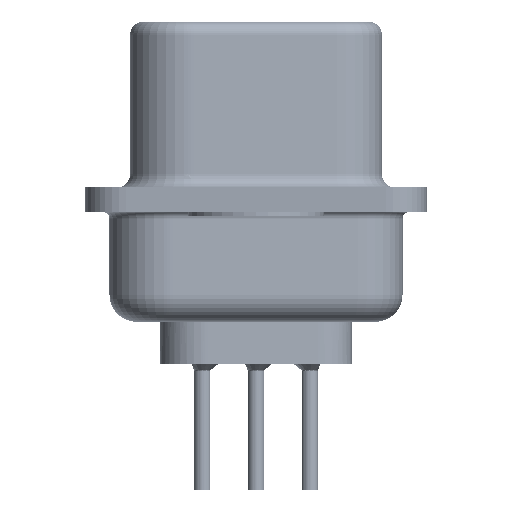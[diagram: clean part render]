
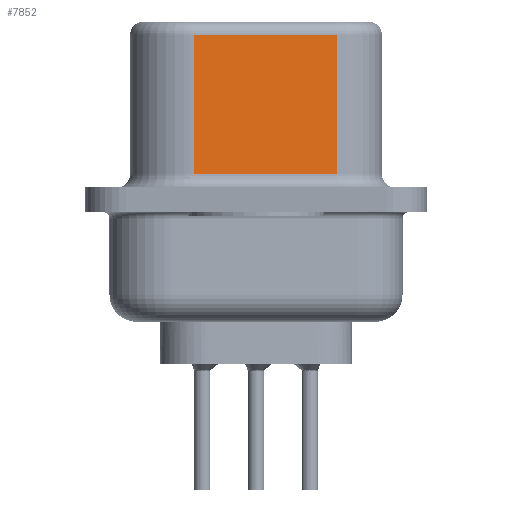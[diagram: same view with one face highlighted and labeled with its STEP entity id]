
A CAD part, left-side view. The second image highlights one B-rep face of the part: STEP entity #7852.
In plain terms, the highlighted planar face has unit normal (-0.985, -0.174, 0).
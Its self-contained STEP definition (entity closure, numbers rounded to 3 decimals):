
#1953 = DIRECTION ( 'NONE',  ( 0., 0., -1. ) ) ;
#3079 = CARTESIAN_POINT ( 'NONE',  ( 4.551, -2.987, 6.07 ) ) ;
#3446 = CARTESIAN_POINT ( 'NONE',  ( 4.551, -2.987, 0.95 ) ) ;
#3955 = LINE ( 'NONE', #13859, #12807 ) ;
#5753 = EDGE_CURVE ( 'NONE', #15745, #7015, #3955, .T. ) ;
#7015 = VERTEX_POINT ( 'NONE', #27484 ) ;
#7018 = ORIENTED_EDGE ( 'NONE', *, *, #5753, .T. ) ;
#7852 = ADVANCED_FACE ( 'NONE', ( #9505 ), #21688, .F. ) ;
#8323 = EDGE_CURVE ( 'NONE', #18790, #12468, #19392, .T. ) ;
#9505 = FACE_OUTER_BOUND ( 'NONE', #10460, .T. ) ;
#9689 = ORIENTED_EDGE ( 'NONE', *, *, #16191, .T. ) ;
#10460 = EDGE_LOOP ( 'NONE', ( #18000, #9689, #7018, #23546 ) ) ;
#11807 = VECTOR ( 'NONE', #1953, 1000. ) ;
#12468 = VERTEX_POINT ( 'NONE', #19099 ) ;
#12769 = AXIS2_PLACEMENT_3D ( 'NONE', #26602, #31407, #28999 ) ;
#12807 = VECTOR ( 'NONE', #30656, 1000. ) ;
#13667 = DIRECTION ( 'NONE',  ( 0.174, -0.985, 0. ) ) ;
#13826 = LINE ( 'NONE', #3446, #20346 ) ;
#13859 = CARTESIAN_POINT ( 'NONE',  ( 3.62, 2.293, 6.57 ) ) ;
#15745 = VERTEX_POINT ( 'NONE', #25020 ) ;
#15763 = VECTOR ( 'NONE', #24688, 1000. ) ;
#16191 = EDGE_CURVE ( 'NONE', #18790, #15745, #24842, .T. ) ;
#18000 = ORIENTED_EDGE ( 'NONE', *, *, #8323, .F. ) ;
#18486 = EDGE_CURVE ( 'NONE', #7015, #12468, #13826, .T. ) ;
#18790 = VERTEX_POINT ( 'NONE', #27411 ) ;
#19099 = CARTESIAN_POINT ( 'NONE',  ( 4.551, -2.987, 0.95 ) ) ;
#19392 = LINE ( 'NONE', #26413, #11807 ) ;
#20346 = VECTOR ( 'NONE', #13667, 1000. ) ;
#21688 = PLANE ( 'NONE',  #12769 ) ;
#23546 = ORIENTED_EDGE ( 'NONE', *, *, #18486, .T. ) ;
#24688 = DIRECTION ( 'NONE',  ( -0.174, 0.985, 0. ) ) ;
#24842 = LINE ( 'NONE', #3079, #15763 ) ;
#25020 = CARTESIAN_POINT ( 'NONE',  ( 3.62, 2.293, 6.07 ) ) ;
#26413 = CARTESIAN_POINT ( 'NONE',  ( 4.551, -2.987, 6.57 ) ) ;
#26602 = CARTESIAN_POINT ( 'NONE',  ( 4.551, -2.987, 6.57 ) ) ;
#27411 = CARTESIAN_POINT ( 'NONE',  ( 4.551, -2.987, 6.07 ) ) ;
#27484 = CARTESIAN_POINT ( 'NONE',  ( 3.62, 2.293, 0.95 ) ) ;
#28999 = DIRECTION ( 'NONE',  ( -0.174, 0.985, 0. ) ) ;
#30656 = DIRECTION ( 'NONE',  ( 0., 0., -1. ) ) ;
#31407 = DIRECTION ( 'NONE',  ( 0.985, 0.174, 0. ) ) ;
